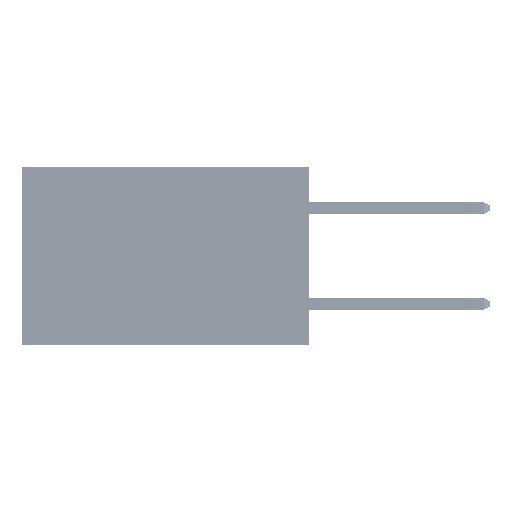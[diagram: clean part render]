
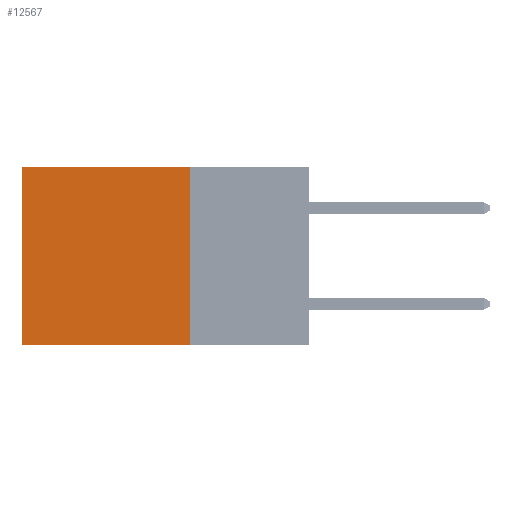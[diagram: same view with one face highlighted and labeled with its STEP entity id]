
A CAD part, left-side view. The second image highlights one B-rep face of the part: STEP entity #12567.
In plain terms, the highlighted planar face has unit normal (-1, 0, 0).
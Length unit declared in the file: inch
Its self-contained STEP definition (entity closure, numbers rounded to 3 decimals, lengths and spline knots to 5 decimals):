
#355 = CARTESIAN_POINT ( 'NONE',  ( 0.2875, 0.25, 0. ) ) ;
#3416 = LINE ( 'NONE', #29739, #4678 ) ;
#4678 = VECTOR ( 'NONE', #32642, 39.37008 ) ;
#4875 = DIRECTION ( 'NONE',  ( 0., 0., -1. ) ) ;
#5028 = DIRECTION ( 'NONE',  ( 0., 1., 0. ) ) ;
#5237 = EDGE_CURVE ( 'NONE', #43366, #16138, #45928, .T. ) ;
#7127 = AXIS2_PLACEMENT_3D ( 'NONE', #355, #15092, #29832 ) ;
#7355 = EDGE_LOOP ( 'NONE', ( #15368, #32180, #34956, #24855 ) ) ;
#8525 = CARTESIAN_POINT ( 'NONE',  ( 0.2875, 0.6, -0.37 ) ) ;
#12567 = ADVANCED_FACE ( 'NONE', ( #26426 ), #33446, .F. ) ;
#12839 = CARTESIAN_POINT ( 'NONE',  ( 0.2875, 0.6, 0. ) ) ;
#14224 = CARTESIAN_POINT ( 'NONE',  ( 0.2875, 0.6, 0. ) ) ;
#15092 = DIRECTION ( 'NONE',  ( 1., 0., 0. ) ) ;
#15368 = ORIENTED_EDGE ( 'NONE', *, *, #5237, .T. ) ;
#16138 = VERTEX_POINT ( 'NONE', #8525 ) ;
#16510 = EDGE_CURVE ( 'NONE', #32717, #43366, #23371, .T. ) ;
#16530 = CARTESIAN_POINT ( 'NONE',  ( 0.2875, 0.25, 0. ) ) ;
#19235 = LINE ( 'NONE', #19709, #29961 ) ;
#19709 = CARTESIAN_POINT ( 'NONE',  ( 0.2875, 0.25, -0.37 ) ) ;
#23371 = LINE ( 'NONE', #23606, #37456 ) ;
#23606 = CARTESIAN_POINT ( 'NONE',  ( 0.2875, 0.25, 0. ) ) ;
#24855 = ORIENTED_EDGE ( 'NONE', *, *, #16510, .T. ) ;
#26426 = FACE_OUTER_BOUND ( 'NONE', #7355, .T. ) ;
#26537 = EDGE_CURVE ( 'NONE', #33810, #16138, #19235, .T. ) ;
#28875 = EDGE_CURVE ( 'NONE', #32717, #33810, #3416, .T. ) ;
#29138 = CARTESIAN_POINT ( 'NONE',  ( 0.2875, 0.25, -0.37 ) ) ;
#29739 = CARTESIAN_POINT ( 'NONE',  ( 0.2875, 0.25, 0. ) ) ;
#29832 = DIRECTION ( 'NONE',  ( 0., 0., -1. ) ) ;
#29961 = VECTOR ( 'NONE', #38551, 39.37008 ) ;
#32180 = ORIENTED_EDGE ( 'NONE', *, *, #26537, .F. ) ;
#32642 = DIRECTION ( 'NONE',  ( 0., 0., -1. ) ) ;
#32717 = VERTEX_POINT ( 'NONE', #16530 ) ;
#33446 = PLANE ( 'NONE',  #7127 ) ;
#33810 = VERTEX_POINT ( 'NONE', #29138 ) ;
#34956 = ORIENTED_EDGE ( 'NONE', *, *, #28875, .F. ) ;
#37456 = VECTOR ( 'NONE', #5028, 39.37008 ) ;
#38551 = DIRECTION ( 'NONE',  ( 0., 1., 0. ) ) ;
#40021 = VECTOR ( 'NONE', #4875, 39.37008 ) ;
#43366 = VERTEX_POINT ( 'NONE', #14224 ) ;
#45928 = LINE ( 'NONE', #12839, #40021 ) ;
